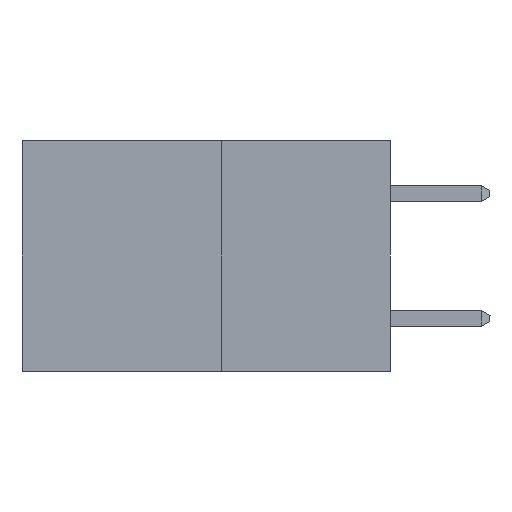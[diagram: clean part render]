
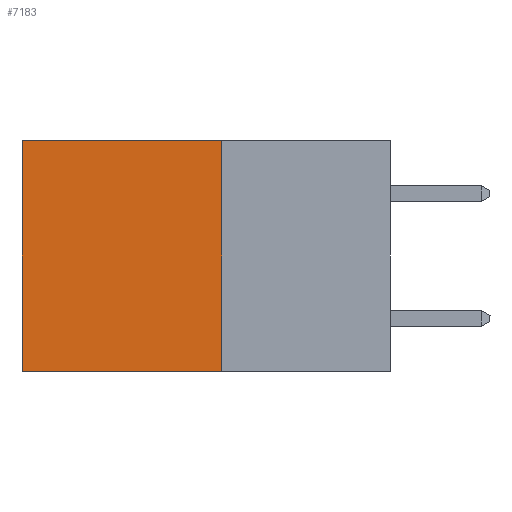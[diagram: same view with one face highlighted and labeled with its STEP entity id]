
A CAD part, left-side view. The second image highlights one B-rep face of the part: STEP entity #7183.
In plain terms, the highlighted planar face has unit normal (-1, 0, 0).
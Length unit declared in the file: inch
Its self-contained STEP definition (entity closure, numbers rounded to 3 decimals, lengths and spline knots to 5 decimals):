
#126 = EDGE_LOOP ( 'NONE', ( #4897, #4644, #5804, #6016 ) ) ;
#230 = LINE ( 'NONE', #5773, #2249 ) ;
#439 = EDGE_CURVE ( 'NONE', #6204, #4620, #5744, .T. ) ;
#703 = EDGE_CURVE ( 'NONE', #4620, #6221, #2733, .T. ) ;
#2162 = AXIS2_PLACEMENT_3D ( 'NONE', #3702, #8746, #4470 ) ;
#2249 = VECTOR ( 'NONE', #9314, 39.37008 ) ;
#2452 = DIRECTION ( 'NONE',  ( 0., 0., -1. ) ) ;
#2733 = LINE ( 'NONE', #8940, #8386 ) ;
#3702 = CARTESIAN_POINT ( 'NONE',  ( 0.277, 0.27, -0.37 ) ) ;
#3745 = CARTESIAN_POINT ( 'NONE',  ( 0.277, 0.27, 0. ) ) ;
#4470 = DIRECTION ( 'NONE',  ( 0., 0., -1. ) ) ;
#4620 = VERTEX_POINT ( 'NONE', #4930 ) ;
#4644 = ORIENTED_EDGE ( 'NONE', *, *, #5927, .F. ) ;
#4897 = ORIENTED_EDGE ( 'NONE', *, *, #703, .T. ) ;
#4930 = CARTESIAN_POINT ( 'NONE',  ( 0.277, 0.59, 0. ) ) ;
#5130 = CARTESIAN_POINT ( 'NONE',  ( 0.277, 0.27, 0. ) ) ;
#5744 = LINE ( 'NONE', #5130, #9262 ) ;
#5773 = CARTESIAN_POINT ( 'NONE',  ( 0.277, 0.27, -0.37 ) ) ;
#5804 = ORIENTED_EDGE ( 'NONE', *, *, #6031, .F. ) ;
#5860 = VECTOR ( 'NONE', #8006, 39.37008 ) ;
#5903 = CARTESIAN_POINT ( 'NONE',  ( 0.277, 0.27, -0.37 ) ) ;
#5927 = EDGE_CURVE ( 'NONE', #8241, #6221, #230, .T. ) ;
#6016 = ORIENTED_EDGE ( 'NONE', *, *, #439, .T. ) ;
#6031 = EDGE_CURVE ( 'NONE', #6204, #8241, #9619, .T. ) ;
#6204 = VERTEX_POINT ( 'NONE', #3745 ) ;
#6221 = VERTEX_POINT ( 'NONE', #8119 ) ;
#7183 = ADVANCED_FACE ( 'NONE', ( #9820 ), #8057, .F. ) ;
#7326 = CARTESIAN_POINT ( 'NONE',  ( 0.277, 0.27, -0.37 ) ) ;
#8006 = DIRECTION ( 'NONE',  ( 0., 0., -1. ) ) ;
#8057 = PLANE ( 'NONE',  #2162 ) ;
#8119 = CARTESIAN_POINT ( 'NONE',  ( 0.277, 0.59, -0.37 ) ) ;
#8206 = DIRECTION ( 'NONE',  ( 0., 1., 0. ) ) ;
#8241 = VERTEX_POINT ( 'NONE', #5903 ) ;
#8386 = VECTOR ( 'NONE', #2452, 39.37008 ) ;
#8746 = DIRECTION ( 'NONE',  ( 1., 0., 0. ) ) ;
#8940 = CARTESIAN_POINT ( 'NONE',  ( 0.277, 0.59, -0.37 ) ) ;
#9262 = VECTOR ( 'NONE', #8206, 39.37008 ) ;
#9314 = DIRECTION ( 'NONE',  ( 0., 1., 0. ) ) ;
#9619 = LINE ( 'NONE', #7326, #5860 ) ;
#9820 = FACE_OUTER_BOUND ( 'NONE', #126, .T. ) ;
